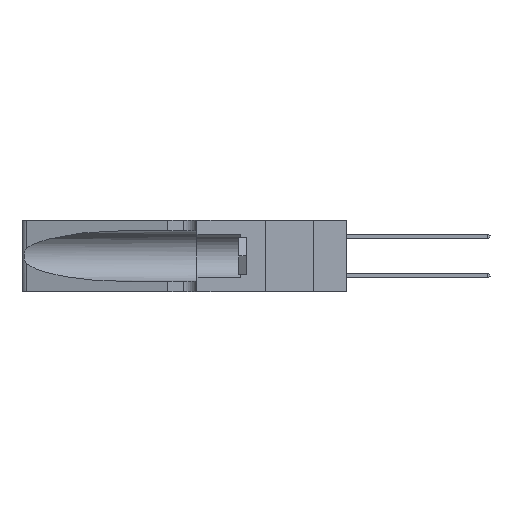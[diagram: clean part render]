
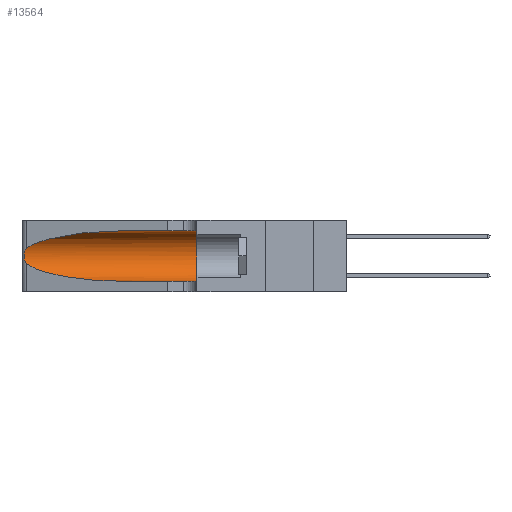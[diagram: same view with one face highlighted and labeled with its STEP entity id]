
A CAD part, left-side view. The second image highlights one B-rep face of the part: STEP entity #13564.
In plain terms, the highlighted cylindrical face has radius 3.308 mm (diameter 6.617 mm), a partial arc.
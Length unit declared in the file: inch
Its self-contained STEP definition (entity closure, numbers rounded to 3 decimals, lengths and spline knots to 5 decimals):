
#72 = CARTESIAN_POINT ( 'NONE',  ( 0.25487, 1.22718, 0.22369 ) ) ;
#85 = CARTESIAN_POINT ( 'NONE',  ( 0.1305, 0.35, 0.05475 ) ) ;
#545 = ORIENTED_EDGE ( 'NONE', *, *, #19794, .F. ) ;
#732 = DIRECTION ( 'NONE',  ( 0., 0., -1. ) ) ;
#1351 = AXIS2_PLACEMENT_3D ( 'NONE', #23218, #4895, #1945 ) ;
#1945 = DIRECTION ( 'NONE',  ( 0., 0., 1. ) ) ;
#2249 = VERTEX_POINT ( 'NONE', #85 ) ;
#2625 = CARTESIAN_POINT ( 'NONE',  ( 0.25487, 1.22718, 0.14631 ) ) ;
#3030 = CARTESIAN_POINT ( 'NONE',  ( 0.1305, 1.61858, 0.05475 ) ) ;
#3063 = CARTESIAN_POINT ( 'NONE',  ( 0.25639, 1.23186, 0.15144 ) ) ;
#3135 = CARTESIAN_POINT ( 'NONE',  ( 0.25487, 1.22718, 0.22369 ) ) ;
#3194 = CARTESIAN_POINT ( 'NONE',  ( 0.26017, 1.23833, 0.17102 ) ) ;
#3877 = EDGE_CURVE ( 'NONE', #38392, #2249, #36211, .T. ) ;
#4895 = DIRECTION ( 'NONE',  ( 0., 1., 0. ) ) ;
#5887 = CARTESIAN_POINT ( 'NONE',  ( 0.25856, 1.23593, 0.16098 ) ) ;
#6024 = ORIENTED_EDGE ( 'NONE', *, *, #25440, .T. ) ;
#6107 = VERTEX_POINT ( 'NONE', #24436 ) ;
#7663 = CYLINDRICAL_SURFACE ( 'NONE', #19784, 0.13025 ) ;
#7807 = ORIENTED_EDGE ( 'NONE', *, *, #33127, .T. ) ;
#8194 = ORIENTED_EDGE ( 'NONE', *, *, #38597, .T. ) ;
#9451 = ORIENTED_EDGE ( 'NONE', *, *, #19318, .T. ) ;
#9688 = CARTESIAN_POINT ( 'NONE',  ( 0.18966, 0.96281, 0.31525 ) ) ;
#10976 = B_SPLINE_CURVE_WITH_KNOTS ( 'NONE', 3,
 ( #72, #15400, #27770, #21517, #12472, #34020, #30849, #33634, #3194, #5887, #15520, #3063, #27620, #24612 ),
 .UNSPECIFIED., .F., .F.,
 ( 4, 2, 2, 2, 2, 2, 4 ),
 ( 0., 0.00027, 0.00053, 0.00107, 0.0016, 0.00187, 0.00214 ),
 .UNSPECIFIED. ) ;
#12006 = VECTOR ( 'NONE', #27247, 39.37008 ) ;
#12109 = CARTESIAN_POINT ( 'NONE',  ( 0.1305, 0.72297, 0.05475 ) ) ;
#12239 = VERTEX_POINT ( 'NONE', #3135 ) ;
#12472 = CARTESIAN_POINT ( 'NONE',  ( 0.25854, 1.2359, 0.20912 ) ) ;
#12555 = LINE ( 'NONE', #3030, #20282 ) ;
#13403 =( BOUNDED_CURVE ( )  B_SPLINE_CURVE ( 3, ( #34289, #9688, #31373, #28415 ),
 .UNSPECIFIED., .F., .T. ) 
 B_SPLINE_CURVE_WITH_KNOTS ( ( 4, 4 ),
 ( 1.5708, 2.84003 ),
 .UNSPECIFIED. ) 
 CURVE ( )  GEOMETRIC_REPRESENTATION_ITEM ( )  RATIONAL_B_SPLINE_CURVE ( ( 1., 0.87, 0.87, 1. ) ) 
 REPRESENTATION_ITEM ( '' )  );
#13564 = ADVANCED_FACE ( 'NONE', ( #27906 ), #7663, .F. ) ;
#15400 = CARTESIAN_POINT ( 'NONE',  ( 0.25555, 1.22994, 0.2215 ) ) ;
#15520 = CARTESIAN_POINT ( 'NONE',  ( 0.25789, 1.23486, 0.15765 ) ) ;
#16654 = CARTESIAN_POINT ( 'NONE',  ( 0.18966, 0.96281, 0.05475 ) ) ;
#19318 = EDGE_CURVE ( 'NONE', #29436, #21920, #23536, .T. ) ;
#19784 = AXIS2_PLACEMENT_3D ( 'NONE', #32036, #31774, #732 ) ;
#19794 = EDGE_CURVE ( 'NONE', #6107, #38392, #32728, .T. ) ;
#19911 = CARTESIAN_POINT ( 'NONE',  ( 0.25487, 1.22718, 0.14631 ) ) ;
#20282 = VECTOR ( 'NONE', #27584, 39.37008 ) ;
#21017 = CARTESIAN_POINT ( 'NONE',  ( 0.1305, 1.61858, 0.31525 ) ) ;
#21517 = CARTESIAN_POINT ( 'NONE',  ( 0.25787, 1.23484, 0.2124 ) ) ;
#21920 = VERTEX_POINT ( 'NONE', #12109 ) ;
#23218 = CARTESIAN_POINT ( 'NONE',  ( 0.1305, 0.35, 0.185 ) ) ;
#23259 = CARTESIAN_POINT ( 'NONE',  ( 0.1305, 0.35, 0.31525 ) ) ;
#23536 =( BOUNDED_CURVE ( )  B_SPLINE_CURVE ( 3, ( #19911, #35108, #16654, #29107 ),
 .UNSPECIFIED., .F., .T. ) 
 B_SPLINE_CURVE_WITH_KNOTS ( ( 4, 4 ),
 ( 3.44316, 4.71239 ),
 .UNSPECIFIED. ) 
 CURVE ( )  GEOMETRIC_REPRESENTATION_ITEM ( )  RATIONAL_B_SPLINE_CURVE ( ( 1., 0.87, 0.87, 1. ) ) 
 REPRESENTATION_ITEM ( '' )  );
#24436 = CARTESIAN_POINT ( 'NONE',  ( 0.1305, 0.72297, 0.31525 ) ) ;
#24612 = CARTESIAN_POINT ( 'NONE',  ( 0.25487, 1.22718, 0.14631 ) ) ;
#25440 = EDGE_CURVE ( 'NONE', #6107, #12239, #13403, .T. ) ;
#27247 = DIRECTION ( 'NONE',  ( 0., -1., 0. ) ) ;
#27584 = DIRECTION ( 'NONE',  ( 0., -1., 0. ) ) ;
#27620 = CARTESIAN_POINT ( 'NONE',  ( 0.25555, 1.22993, 0.14849 ) ) ;
#27676 = EDGE_LOOP ( 'NONE', ( #6024, #8194, #9451, #7807, #38880, #545 ) ) ;
#27770 = CARTESIAN_POINT ( 'NONE',  ( 0.25639, 1.23184, 0.21858 ) ) ;
#27906 = FACE_OUTER_BOUND ( 'NONE', #27676, .T. ) ;
#28415 = CARTESIAN_POINT ( 'NONE',  ( 0.25487, 1.22718, 0.22369 ) ) ;
#29107 = CARTESIAN_POINT ( 'NONE',  ( 0.1305, 0.72297, 0.05475 ) ) ;
#29436 = VERTEX_POINT ( 'NONE', #2625 ) ;
#30849 = CARTESIAN_POINT ( 'NONE',  ( 0.26075, 1.23896, 0.19203 ) ) ;
#31373 = CARTESIAN_POINT ( 'NONE',  ( 0.2373, 1.15595, 0.28018 ) ) ;
#31774 = DIRECTION ( 'NONE',  ( 0., -1., 0. ) ) ;
#32036 = CARTESIAN_POINT ( 'NONE',  ( 0.1305, 1.61858, 0.185 ) ) ;
#32728 = LINE ( 'NONE', #21017, #12006 ) ;
#33127 = EDGE_CURVE ( 'NONE', #21920, #2249, #12555, .T. ) ;
#33634 = CARTESIAN_POINT ( 'NONE',  ( 0.26075, 1.23896, 0.178 ) ) ;
#34020 = CARTESIAN_POINT ( 'NONE',  ( 0.26018, 1.23835, 0.19895 ) ) ;
#34289 = CARTESIAN_POINT ( 'NONE',  ( 0.1305, 0.72297, 0.31525 ) ) ;
#35108 = CARTESIAN_POINT ( 'NONE',  ( 0.2373, 1.15595, 0.08982 ) ) ;
#36211 = CIRCLE ( 'NONE', #1351, 0.13025 ) ;
#38392 = VERTEX_POINT ( 'NONE', #23259 ) ;
#38597 = EDGE_CURVE ( 'NONE', #12239, #29436, #10976, .T. ) ;
#38880 = ORIENTED_EDGE ( 'NONE', *, *, #3877, .F. ) ;
